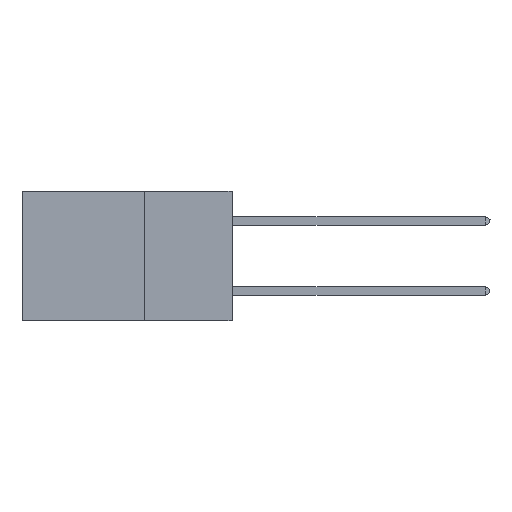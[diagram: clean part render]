
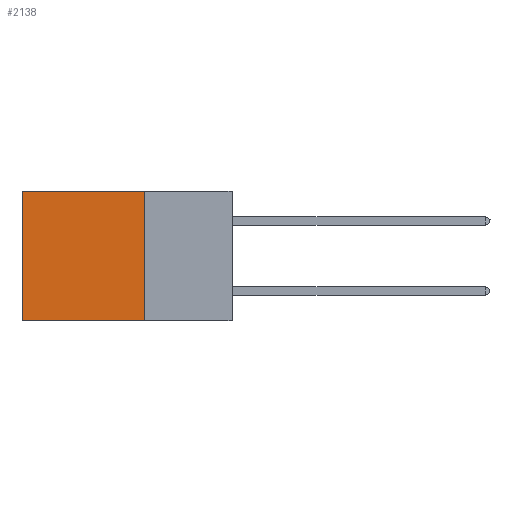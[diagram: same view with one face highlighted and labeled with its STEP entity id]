
A CAD part, left-side view. The second image highlights one B-rep face of the part: STEP entity #2138.
In plain terms, the highlighted planar face has unit normal (-1, 0, 0).
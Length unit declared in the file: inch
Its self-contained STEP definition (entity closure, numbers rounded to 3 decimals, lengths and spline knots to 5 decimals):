
#1396 = EDGE_CURVE ( 'NONE', #3363, #26688, #5561, .T. ) ;
#2138 = ADVANCED_FACE ( 'NONE', ( #15329 ), #25973, .F. ) ;
#3363 = VERTEX_POINT ( 'NONE', #10872 ) ;
#3686 = VECTOR ( 'NONE', #25646, 39.37008 ) ;
#4073 = CARTESIAN_POINT ( 'NONE',  ( 0.2875, 0.25, 0. ) ) ;
#5561 = LINE ( 'NONE', #4073, #12308 ) ;
#7231 = CARTESIAN_POINT ( 'NONE',  ( 0.2875, 0.6, 0. ) ) ;
#7262 = DIRECTION ( 'NONE',  ( 1., 0., 0. ) ) ;
#8986 = LINE ( 'NONE', #17302, #3686 ) ;
#9357 = CARTESIAN_POINT ( 'NONE',  ( 0.2875, 0.25, -0.37 ) ) ;
#9839 = VERTEX_POINT ( 'NONE', #20727 ) ;
#10123 = EDGE_CURVE ( 'NONE', #3363, #9839, #8986, .T. ) ;
#10872 = CARTESIAN_POINT ( 'NONE',  ( 0.2875, 0.25, 0. ) ) ;
#12308 = VECTOR ( 'NONE', #26826, 39.37008 ) ;
#12911 = ORIENTED_EDGE ( 'NONE', *, *, #15352, .F. ) ;
#13586 = EDGE_CURVE ( 'NONE', #26688, #15200, #14964, .T. ) ;
#14705 = VECTOR ( 'NONE', #23836, 39.37008 ) ;
#14964 = LINE ( 'NONE', #18644, #22479 ) ;
#15200 = VERTEX_POINT ( 'NONE', #20700 ) ;
#15223 = ORIENTED_EDGE ( 'NONE', *, *, #10123, .F. ) ;
#15329 = FACE_OUTER_BOUND ( 'NONE', #16534, .T. ) ;
#15352 = EDGE_CURVE ( 'NONE', #9839, #15200, #22050, .T. ) ;
#15587 = DIRECTION ( 'NONE',  ( 0., 0., -1. ) ) ;
#16534 = EDGE_LOOP ( 'NONE', ( #23512, #12911, #15223, #17552 ) ) ;
#16596 = DIRECTION ( 'NONE',  ( 0., 0., -1. ) ) ;
#17302 = CARTESIAN_POINT ( 'NONE',  ( 0.2875, 0.25, 0. ) ) ;
#17552 = ORIENTED_EDGE ( 'NONE', *, *, #1396, .T. ) ;
#18644 = CARTESIAN_POINT ( 'NONE',  ( 0.2875, 0.6, 0. ) ) ;
#20700 = CARTESIAN_POINT ( 'NONE',  ( 0.2875, 0.6, -0.37 ) ) ;
#20727 = CARTESIAN_POINT ( 'NONE',  ( 0.2875, 0.25, -0.37 ) ) ;
#21333 = CARTESIAN_POINT ( 'NONE',  ( 0.2875, 0.25, 0. ) ) ;
#21486 = AXIS2_PLACEMENT_3D ( 'NONE', #21333, #7262, #15587 ) ;
#22050 = LINE ( 'NONE', #9357, #14705 ) ;
#22479 = VECTOR ( 'NONE', #16596, 39.37008 ) ;
#23512 = ORIENTED_EDGE ( 'NONE', *, *, #13586, .T. ) ;
#23836 = DIRECTION ( 'NONE',  ( 0., 1., 0. ) ) ;
#25646 = DIRECTION ( 'NONE',  ( 0., 0., -1. ) ) ;
#25973 = PLANE ( 'NONE',  #21486 ) ;
#26688 = VERTEX_POINT ( 'NONE', #7231 ) ;
#26826 = DIRECTION ( 'NONE',  ( 0., 1., 0. ) ) ;
